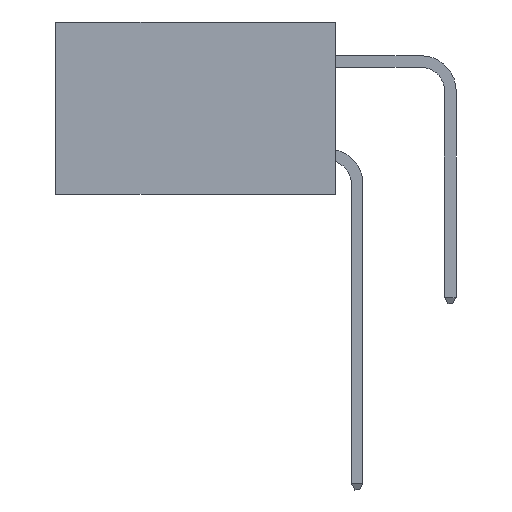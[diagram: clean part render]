
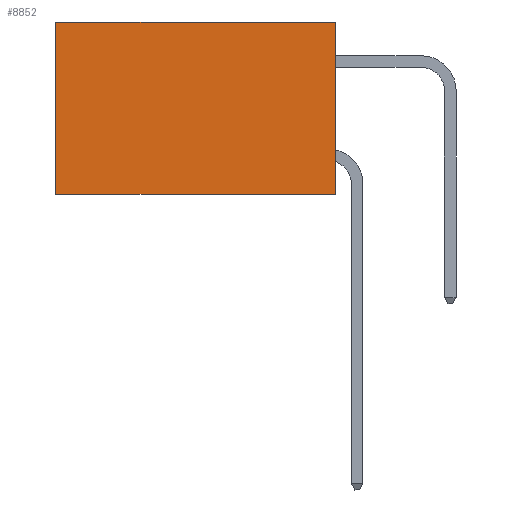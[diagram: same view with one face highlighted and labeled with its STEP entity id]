
A CAD part, left-side view. The second image highlights one B-rep face of the part: STEP entity #8852.
In plain terms, the highlighted planar face has unit normal (-1, 0, 0).
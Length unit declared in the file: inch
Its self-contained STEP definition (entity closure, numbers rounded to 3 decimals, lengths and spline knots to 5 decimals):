
#278 = DIRECTION ( 'NONE',  ( 0., 0., -1. ) ) ;
#290 = DIRECTION ( 'NONE',  ( 1., 0., 0. ) ) ;
#313 = PLANE ( 'NONE',  #5099 ) ;
#414 = CARTESIAN_POINT ( 'NONE',  ( 0.2875, 0., 0. ) ) ;
#728 = VECTOR ( 'NONE', #4428, 39.37008 ) ;
#1088 = EDGE_LOOP ( 'NONE', ( #6982, #12779, #12335, #2230 ) ) ;
#1536 = EDGE_CURVE ( 'NONE', #4177, #5634, #7094, .T. ) ;
#1730 = CARTESIAN_POINT ( 'NONE',  ( 0.2875, 0., -0.37 ) ) ;
#2230 = ORIENTED_EDGE ( 'NONE', *, *, #15903, .T. ) ;
#2526 = FACE_OUTER_BOUND ( 'NONE', #1088, .T. ) ;
#2752 = CARTESIAN_POINT ( 'NONE',  ( 0.2875, 0., 0. ) ) ;
#3923 = CARTESIAN_POINT ( 'NONE',  ( 0.2875, 0.6, -0.37 ) ) ;
#4109 = LINE ( 'NONE', #4467, #728 ) ;
#4177 = VERTEX_POINT ( 'NONE', #2752 ) ;
#4428 = DIRECTION ( 'NONE',  ( 0., 1., 0. ) ) ;
#4467 = CARTESIAN_POINT ( 'NONE',  ( 0.2875, 0., -0.37 ) ) ;
#5099 = AXIS2_PLACEMENT_3D ( 'NONE', #414, #290, #278 ) ;
#5110 = CARTESIAN_POINT ( 'NONE',  ( 0.2875, 0.6, 0. ) ) ;
#5472 = VECTOR ( 'NONE', #6822, 39.37008 ) ;
#5543 = CARTESIAN_POINT ( 'NONE',  ( 0.2875, 0., 0. ) ) ;
#5634 = VERTEX_POINT ( 'NONE', #1730 ) ;
#6822 = DIRECTION ( 'NONE',  ( 0., 1., 0. ) ) ;
#6982 = ORIENTED_EDGE ( 'NONE', *, *, #12626, .T. ) ;
#7094 = LINE ( 'NONE', #8839, #9994 ) ;
#7189 = EDGE_CURVE ( 'NONE', #5634, #11232, #4109, .T. ) ;
#8495 = DIRECTION ( 'NONE',  ( 0., 0., -1. ) ) ;
#8798 = LINE ( 'NONE', #5543, #5472 ) ;
#8839 = CARTESIAN_POINT ( 'NONE',  ( 0.2875, 0., 0. ) ) ;
#8852 = ADVANCED_FACE ( 'NONE', ( #2526 ), #313, .F. ) ;
#8936 = DIRECTION ( 'NONE',  ( 0., 0., -1. ) ) ;
#9692 = VECTOR ( 'NONE', #8495, 39.37008 ) ;
#9994 = VECTOR ( 'NONE', #8936, 39.37008 ) ;
#11232 = VERTEX_POINT ( 'NONE', #3923 ) ;
#12335 = ORIENTED_EDGE ( 'NONE', *, *, #1536, .F. ) ;
#12626 = EDGE_CURVE ( 'NONE', #14025, #11232, #15749, .T. ) ;
#12779 = ORIENTED_EDGE ( 'NONE', *, *, #7189, .F. ) ;
#14025 = VERTEX_POINT ( 'NONE', #5110 ) ;
#14571 = CARTESIAN_POINT ( 'NONE',  ( 0.2875, 0.6, 0. ) ) ;
#15749 = LINE ( 'NONE', #14571, #9692 ) ;
#15903 = EDGE_CURVE ( 'NONE', #4177, #14025, #8798, .T. ) ;
